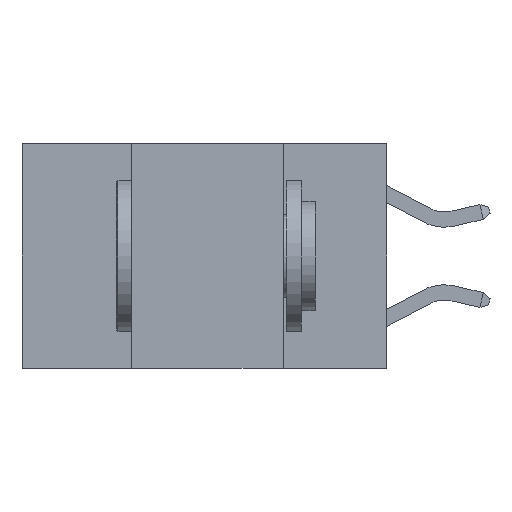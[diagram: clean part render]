
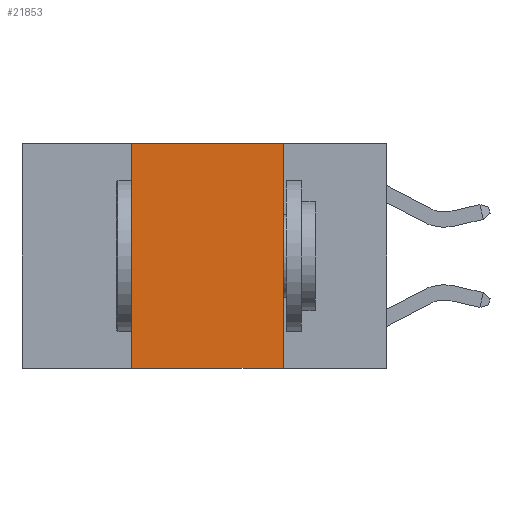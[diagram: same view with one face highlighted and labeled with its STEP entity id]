
A CAD part, left-side view. The second image highlights one B-rep face of the part: STEP entity #21853.
In plain terms, the highlighted planar face has unit normal (-1, 0, 0).
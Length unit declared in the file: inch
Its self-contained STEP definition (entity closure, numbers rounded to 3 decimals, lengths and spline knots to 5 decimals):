
#1374 = DIRECTION ( 'NONE',  ( 0., 0., 1. ) ) ;
#2843 = ORIENTED_EDGE ( 'NONE', *, *, #15630, .F. ) ;
#3732 = PLANE ( 'NONE',  #18315 ) ;
#4383 = VECTOR ( 'NONE', #9520, 39.37008 ) ;
#4902 = CARTESIAN_POINT ( 'NONE',  ( 0., 0.6, 0. ) ) ;
#5531 = EDGE_LOOP ( 'NONE', ( #2843, #25627, #9120, #25447 ) ) ;
#6688 = DIRECTION ( 'NONE',  ( 0., 0., -1. ) ) ;
#7964 = CARTESIAN_POINT ( 'NONE',  ( 0., 0.42, -0.37 ) ) ;
#8091 = CARTESIAN_POINT ( 'NONE',  ( 0., 0.17, -0.37 ) ) ;
#9120 = ORIENTED_EDGE ( 'NONE', *, *, #18524, .F. ) ;
#9316 = CARTESIAN_POINT ( 'NONE',  ( 0., 0.6, 0. ) ) ;
#9520 = DIRECTION ( 'NONE',  ( 0., -1., 0. ) ) ;
#9579 = DIRECTION ( 'NONE',  ( 1., 0., 0. ) ) ;
#9841 = VERTEX_POINT ( 'NONE', #7964 ) ;
#10561 = LINE ( 'NONE', #10697, #24487 ) ;
#10697 = CARTESIAN_POINT ( 'NONE',  ( 0., 0.17, 0. ) ) ;
#12169 = VECTOR ( 'NONE', #23269, 39.37008 ) ;
#14823 = EDGE_CURVE ( 'NONE', #19750, #16500, #16626, .T. ) ;
#15537 = LINE ( 'NONE', #23642, #4383 ) ;
#15630 = EDGE_CURVE ( 'NONE', #16500, #20429, #10561, .T. ) ;
#16500 = VERTEX_POINT ( 'NONE', #22355 ) ;
#16626 = LINE ( 'NONE', #4902, #12169 ) ;
#18315 = AXIS2_PLACEMENT_3D ( 'NONE', #9316, #9579, #25694 ) ;
#18524 = EDGE_CURVE ( 'NONE', #9841, #19750, #19216, .T. ) ;
#19216 = LINE ( 'NONE', #25457, #21592 ) ;
#19750 = VERTEX_POINT ( 'NONE', #24714 ) ;
#20429 = VERTEX_POINT ( 'NONE', #8091 ) ;
#21592 = VECTOR ( 'NONE', #1374, 39.37008 ) ;
#21853 = ADVANCED_FACE ( 'NONE', ( #21970 ), #3732, .F. ) ;
#21970 = FACE_OUTER_BOUND ( 'NONE', #5531, .T. ) ;
#22355 = CARTESIAN_POINT ( 'NONE',  ( 0., 0.17, 0. ) ) ;
#23269 = DIRECTION ( 'NONE',  ( 0., -1., 0. ) ) ;
#23642 = CARTESIAN_POINT ( 'NONE',  ( 0., 0.6, -0.37 ) ) ;
#24238 = EDGE_CURVE ( 'NONE', #9841, #20429, #15537, .T. ) ;
#24487 = VECTOR ( 'NONE', #6688, 39.37008 ) ;
#24714 = CARTESIAN_POINT ( 'NONE',  ( 0., 0.42, 0. ) ) ;
#25447 = ORIENTED_EDGE ( 'NONE', *, *, #24238, .T. ) ;
#25457 = CARTESIAN_POINT ( 'NONE',  ( 0., 0.42, 0. ) ) ;
#25627 = ORIENTED_EDGE ( 'NONE', *, *, #14823, .F. ) ;
#25694 = DIRECTION ( 'NONE',  ( 0., 0., -1. ) ) ;
